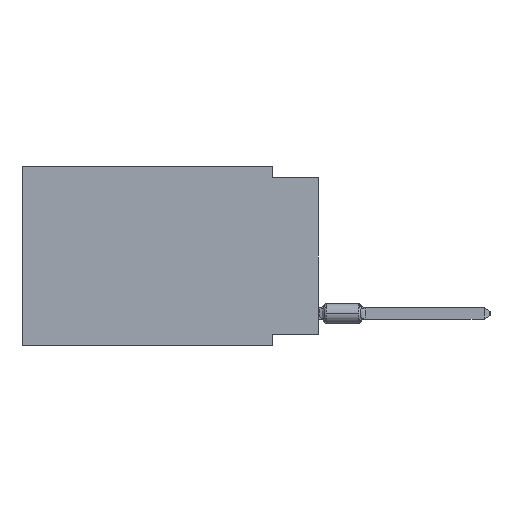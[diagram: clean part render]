
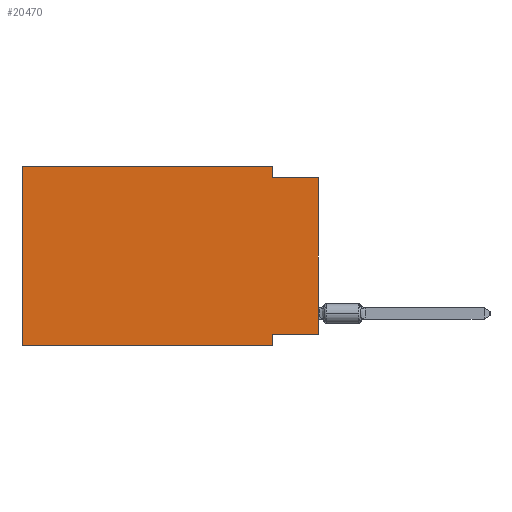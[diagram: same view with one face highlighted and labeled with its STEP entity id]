
A CAD part, left-side view. The second image highlights one B-rep face of the part: STEP entity #20470.
In plain terms, the highlighted planar face has unit normal (-1, 0, 0).
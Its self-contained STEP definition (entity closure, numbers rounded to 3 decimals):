
#256 = VECTOR ( 'NONE', #55127, 1000. ) ;
#718 = VECTOR ( 'NONE', #51140, 1000. ) ;
#2230 = LINE ( 'NONE', #23503, #9492 ) ;
#2526 = EDGE_CURVE ( 'NONE', #50801, #5310, #46599, .T. ) ;
#3283 = ORIENTED_EDGE ( 'NONE', *, *, #2526, .F. ) ;
#3721 = CARTESIAN_POINT ( 'NONE',  ( 0., 16.383, 0. ) ) ;
#4202 = CARTESIAN_POINT ( 'NONE',  ( 0., 2.54, -0.635 ) ) ;
#4316 = CARTESIAN_POINT ( 'NONE',  ( 0., 0., -9.271 ) ) ;
#4790 = CARTESIAN_POINT ( 'NONE',  ( 0., 2.54, 0. ) ) ;
#5310 = VERTEX_POINT ( 'NONE', #4790 ) ;
#5397 = DIRECTION ( 'NONE',  ( 1., 0., 0. ) ) ;
#5994 = LINE ( 'NONE', #33183, #256 ) ;
#6272 = DIRECTION ( 'NONE',  ( 0., 0., 1. ) ) ;
#7479 = VERTEX_POINT ( 'NONE', #4202 ) ;
#7527 = VERTEX_POINT ( 'NONE', #46404 ) ;
#9492 = VECTOR ( 'NONE', #44768, 1000. ) ;
#9696 = CARTESIAN_POINT ( 'NONE',  ( 0., 0., -9.271 ) ) ;
#11244 = CARTESIAN_POINT ( 'NONE',  ( 0., 2.54, -9.906 ) ) ;
#12171 = VERTEX_POINT ( 'NONE', #50616 ) ;
#12901 = EDGE_CURVE ( 'NONE', #5310, #7479, #2230, .T. ) ;
#13396 = CARTESIAN_POINT ( 'NONE',  ( 0., 2.54, -9.906 ) ) ;
#13741 = DIRECTION ( 'NONE',  ( 0., -1., 0. ) ) ;
#14072 = DIRECTION ( 'NONE',  ( 0., 0., -1. ) ) ;
#15155 = FACE_OUTER_BOUND ( 'NONE', #34724, .T. ) ;
#17614 = VERTEX_POINT ( 'NONE', #9696 ) ;
#18021 = DIRECTION ( 'NONE',  ( 0., -1., 0. ) ) ;
#18728 = VECTOR ( 'NONE', #13741, 1000. ) ;
#18810 = VECTOR ( 'NONE', #14072, 1000. ) ;
#20470 = ADVANCED_FACE ( 'NONE', ( #15155 ), #58042, .F. ) ;
#23503 = CARTESIAN_POINT ( 'NONE',  ( 0., 2.54, 0. ) ) ;
#24228 = CARTESIAN_POINT ( 'NONE',  ( 0., 16.383, -9.906 ) ) ;
#25097 = ORIENTED_EDGE ( 'NONE', *, *, #33891, .T. ) ;
#25590 = DIRECTION ( 'NONE',  ( 0., 1., 0. ) ) ;
#27021 = ORIENTED_EDGE ( 'NONE', *, *, #50973, .T. ) ;
#28237 = LINE ( 'NONE', #64822, #65533 ) ;
#31388 = AXIS2_PLACEMENT_3D ( 'NONE', #36463, #5397, #32240 ) ;
#32240 = DIRECTION ( 'NONE',  ( 0., 0., -1. ) ) ;
#33183 = CARTESIAN_POINT ( 'NONE',  ( 0., 0., 0. ) ) ;
#33299 = VECTOR ( 'NONE', #18021, 1000. ) ;
#33891 = EDGE_CURVE ( 'NONE', #7527, #62485, #38857, .T. ) ;
#34243 = EDGE_CURVE ( 'NONE', #7527, #50801, #28237, .T. ) ;
#34724 = EDGE_LOOP ( 'NONE', ( #27021, #49476, #34850, #3283, #65319, #25097, #67165, #50146 ) ) ;
#34794 = EDGE_CURVE ( 'NONE', #7479, #67784, #56715, .T. ) ;
#34850 = ORIENTED_EDGE ( 'NONE', *, *, #12901, .F. ) ;
#35724 = LINE ( 'NONE', #13396, #18810 ) ;
#36463 = CARTESIAN_POINT ( 'NONE',  ( 0., 16.383, 0. ) ) ;
#38857 = LINE ( 'NONE', #24228, #18728 ) ;
#41666 = CARTESIAN_POINT ( 'NONE',  ( 0., 0., -0.635 ) ) ;
#41674 = VECTOR ( 'NONE', #25590, 1000. ) ;
#42682 = EDGE_CURVE ( 'NONE', #17614, #12171, #52058, .T. ) ;
#44768 = DIRECTION ( 'NONE',  ( 0., 0., -1. ) ) ;
#46404 = CARTESIAN_POINT ( 'NONE',  ( 0., 16.383, -9.906 ) ) ;
#46599 = LINE ( 'NONE', #3721, #718 ) ;
#49476 = ORIENTED_EDGE ( 'NONE', *, *, #34794, .F. ) ;
#50146 = ORIENTED_EDGE ( 'NONE', *, *, #42682, .F. ) ;
#50616 = CARTESIAN_POINT ( 'NONE',  ( 0., 2.54, -9.271 ) ) ;
#50801 = VERTEX_POINT ( 'NONE', #60351 ) ;
#50973 = EDGE_CURVE ( 'NONE', #17614, #67784, #5994, .T. ) ;
#51140 = DIRECTION ( 'NONE',  ( 0., -1., 0. ) ) ;
#52058 = LINE ( 'NONE', #4316, #41674 ) ;
#55127 = DIRECTION ( 'NONE',  ( 0., 0., 1. ) ) ;
#56715 = LINE ( 'NONE', #65788, #33299 ) ;
#57837 = EDGE_CURVE ( 'NONE', #12171, #62485, #35724, .T. ) ;
#58042 = PLANE ( 'NONE',  #31388 ) ;
#60351 = CARTESIAN_POINT ( 'NONE',  ( 0., 16.383, 0. ) ) ;
#62485 = VERTEX_POINT ( 'NONE', #11244 ) ;
#64822 = CARTESIAN_POINT ( 'NONE',  ( 0., 16.383, 0. ) ) ;
#65319 = ORIENTED_EDGE ( 'NONE', *, *, #34243, .F. ) ;
#65533 = VECTOR ( 'NONE', #6272, 1000. ) ;
#65788 = CARTESIAN_POINT ( 'NONE',  ( 0., 0., -0.635 ) ) ;
#67165 = ORIENTED_EDGE ( 'NONE', *, *, #57837, .F. ) ;
#67784 = VERTEX_POINT ( 'NONE', #41666 ) ;
